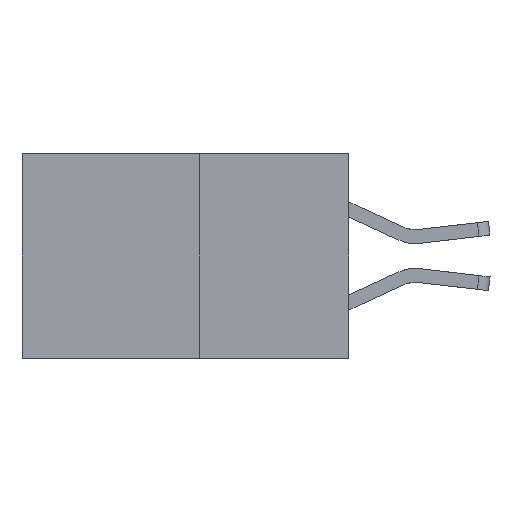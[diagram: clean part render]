
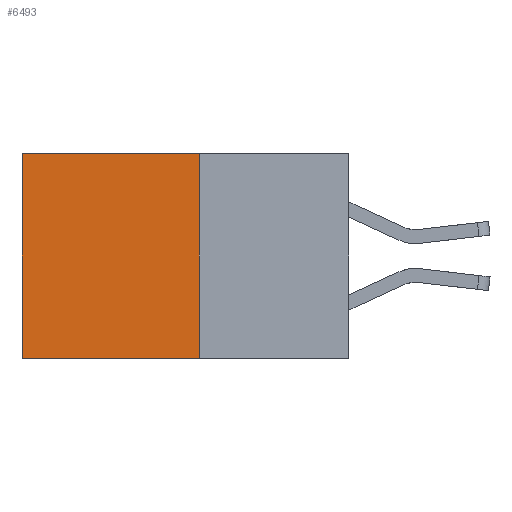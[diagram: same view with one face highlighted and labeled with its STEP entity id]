
A CAD part, left-side view. The second image highlights one B-rep face of the part: STEP entity #6493.
In plain terms, the highlighted planar face has unit normal (-1, 0, 0).
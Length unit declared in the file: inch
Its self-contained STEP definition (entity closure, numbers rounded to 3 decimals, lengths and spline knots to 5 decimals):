
#88 = VERTEX_POINT ( 'NONE', #8631 ) ;
#135 = VERTEX_POINT ( 'NONE', #5107 ) ;
#178 = AXIS2_PLACEMENT_3D ( 'NONE', #1189, #1177, #1162 ) ;
#460 = EDGE_CURVE ( 'NONE', #7870, #88, #4720, .T. ) ;
#564 = EDGE_CURVE ( 'NONE', #88, #135, #7723, .T. ) ;
#948 = VECTOR ( 'NONE', #6760, 39.37008 ) ;
#1042 = EDGE_LOOP ( 'NONE', ( #2238, #2740, #8108, #6038 ) ) ;
#1087 = CARTESIAN_POINT ( 'NONE',  ( 0.277, 0.27, 0. ) ) ;
#1162 = DIRECTION ( 'NONE',  ( 0., 0., -1. ) ) ;
#1177 = DIRECTION ( 'NONE',  ( 1., 0., 0. ) ) ;
#1189 = CARTESIAN_POINT ( 'NONE',  ( 0.277, 0.27, -0.37 ) ) ;
#1464 = PLANE ( 'NONE',  #178 ) ;
#1886 = CARTESIAN_POINT ( 'NONE',  ( 0.277, 0.27, 0. ) ) ;
#1914 = LINE ( 'NONE', #6592, #6076 ) ;
#1982 = DIRECTION ( 'NONE',  ( 0., 1., 0. ) ) ;
#2068 = CARTESIAN_POINT ( 'NONE',  ( 0.277, 0.27, -0.37 ) ) ;
#2238 = ORIENTED_EDGE ( 'NONE', *, *, #5603, .T. ) ;
#2740 = ORIENTED_EDGE ( 'NONE', *, *, #564, .F. ) ;
#3786 = CARTESIAN_POINT ( 'NONE',  ( 0.277, 0.59, 0. ) ) ;
#4577 = LINE ( 'NONE', #1886, #6619 ) ;
#4720 = LINE ( 'NONE', #6974, #8740 ) ;
#4922 = DIRECTION ( 'NONE',  ( 0., 0., -1. ) ) ;
#5107 = CARTESIAN_POINT ( 'NONE',  ( 0.277, 0.59, -0.37 ) ) ;
#5603 = EDGE_CURVE ( 'NONE', #7447, #135, #1914, .T. ) ;
#6038 = ORIENTED_EDGE ( 'NONE', *, *, #9775, .T. ) ;
#6076 = VECTOR ( 'NONE', #6689, 39.37008 ) ;
#6493 = ADVANCED_FACE ( 'NONE', ( #10330 ), #1464, .F. ) ;
#6592 = CARTESIAN_POINT ( 'NONE',  ( 0.277, 0.59, -0.37 ) ) ;
#6619 = VECTOR ( 'NONE', #1982, 39.37008 ) ;
#6689 = DIRECTION ( 'NONE',  ( 0., 0., -1. ) ) ;
#6760 = DIRECTION ( 'NONE',  ( 0., 1., 0. ) ) ;
#6974 = CARTESIAN_POINT ( 'NONE',  ( 0.277, 0.27, -0.37 ) ) ;
#7447 = VERTEX_POINT ( 'NONE', #3786 ) ;
#7723 = LINE ( 'NONE', #2068, #948 ) ;
#7870 = VERTEX_POINT ( 'NONE', #1087 ) ;
#8108 = ORIENTED_EDGE ( 'NONE', *, *, #460, .F. ) ;
#8631 = CARTESIAN_POINT ( 'NONE',  ( 0.277, 0.27, -0.37 ) ) ;
#8740 = VECTOR ( 'NONE', #4922, 39.37008 ) ;
#9775 = EDGE_CURVE ( 'NONE', #7870, #7447, #4577, .T. ) ;
#10330 = FACE_OUTER_BOUND ( 'NONE', #1042, .T. ) ;
